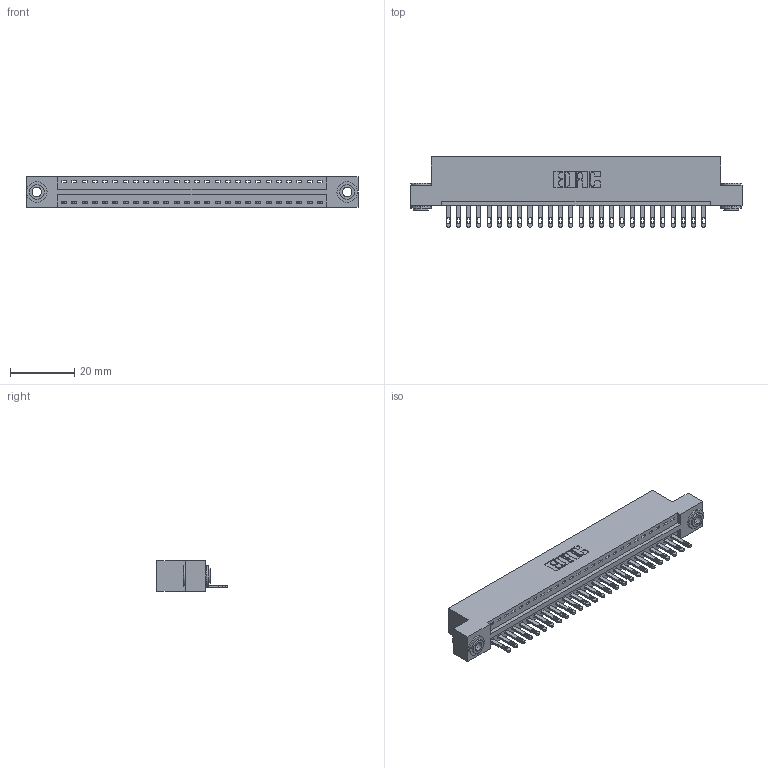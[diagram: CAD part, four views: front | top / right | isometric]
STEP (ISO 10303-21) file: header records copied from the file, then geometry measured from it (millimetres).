
FILE_DESCRIPTION (( 'STEP AP203' ), '1' );
FILE_NAME ('346-026-500-103.STEP', '2022-05-06T01:47:22', ( '' ), ( '' ), 'SwSTEP 2.0', 'SolidWorks 2020', '' );
FILE_SCHEMA (( 'CONFIG_CONTROL_DESIGN' ));
Length unit declared in the file: inch
Products named in the file (4): 345-250-002_345-250-002-102; 346-026-500-103; 345-292-001_345-293-100; 346 Part_Flush Mounting Lugs - 0.156 Dia-TH
Assembly tree (29 placements, depth 2):
  346-026-500-103
    346 Part_Flush Mounting Lugs - 0.156 Dia-TH
    345-292-001_345-293-100  x26
    345-250-002_345-250-002-102  x2
Bounding box: 103.12 x 21.84 x 9.4 mm (x, y, z)
Volume: 9778.4 mm3; surface area: 12361.1 mm2
Topology: 29 solids, 29 shells, 1578 faces, 4809 edges, 3202 vertices
Faces by surface type: plane 984, cylinder 586, cone 8
Entity records: 19286 total; most frequent: CARTESIAN_POINT 3291, ORIENTED_EDGE 3242, DIRECTION 2955, EDGE_CURVE 1621, LINE 1357, VECTOR 1357, VERTEX_POINT 1078, AXIS2_PLACEMENT_3D 799
